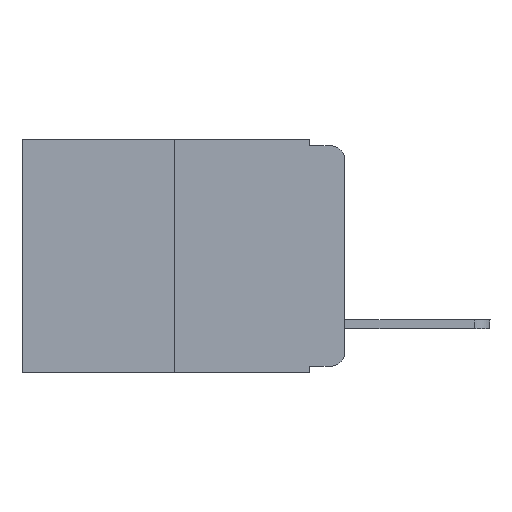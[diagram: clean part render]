
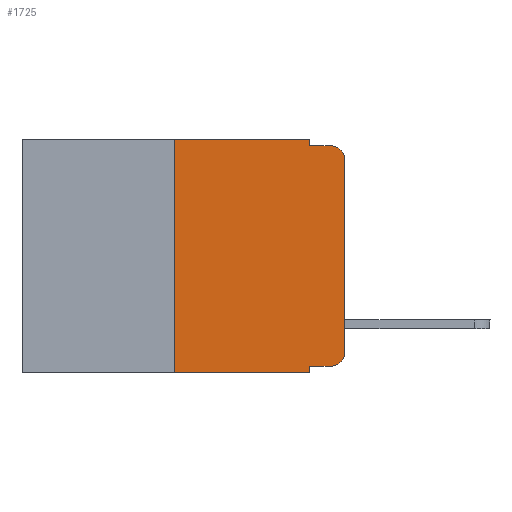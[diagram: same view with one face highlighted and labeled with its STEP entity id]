
A CAD part, left-side view. The second image highlights one B-rep face of the part: STEP entity #1725.
In plain terms, the highlighted planar face has unit normal (-1, 0, 0).
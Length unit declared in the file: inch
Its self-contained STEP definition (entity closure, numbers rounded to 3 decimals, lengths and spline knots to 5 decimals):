
#99 = EDGE_CURVE ( 'NONE', #9774, #3113, #4630, .T. ) ;
#187 = DIRECTION ( 'NONE',  ( 0., 0., 1. ) ) ;
#196 = DIRECTION ( 'NONE',  ( 0., 0., -1. ) ) ;
#486 = VECTOR ( 'NONE', #4476, 39.37008 ) ;
#588 = DIRECTION ( 'NONE',  ( 1., 0., 0. ) ) ;
#628 = DIRECTION ( 'NONE',  ( 0., -1., 0. ) ) ;
#664 = DIRECTION ( 'NONE',  ( 0., -1., 0. ) ) ;
#666 = ORIENTED_EDGE ( 'NONE', *, *, #4712, .T. ) ;
#962 = DIRECTION ( 'NONE',  ( -1., 0., 0. ) ) ;
#1232 = VECTOR ( 'NONE', #664, 39.37008 ) ;
#1253 = EDGE_CURVE ( 'NONE', #8522, #6959, #6556, .T. ) ;
#1318 = LINE ( 'NONE', #5188, #9555 ) ;
#1461 = VECTOR ( 'NONE', #628, 39.37008 ) ;
#1607 = VECTOR ( 'NONE', #8382, 39.37008 ) ;
#1681 = AXIS2_PLACEMENT_3D ( 'NONE', #4606, #588, #6903 ) ;
#1701 = EDGE_CURVE ( 'NONE', #6707, #2656, #3831, .T. ) ;
#1725 = ADVANCED_FACE ( 'NONE', ( #8867 ), #3811, .F. ) ;
#1744 = CARTESIAN_POINT ( 'NONE',  ( 0., 0.02, -0.03 ) ) ;
#2026 = ORIENTED_EDGE ( 'NONE', *, *, #7858, .F. ) ;
#2173 = VERTEX_POINT ( 'NONE', #7969 ) ;
#2255 = ORIENTED_EDGE ( 'NONE', *, *, #3252, .T. ) ;
#2523 = ORIENTED_EDGE ( 'NONE', *, *, #4235, .F. ) ;
#2622 = DIRECTION ( 'NONE',  ( 0., 0., -1. ) ) ;
#2656 = VERTEX_POINT ( 'NONE', #4890 ) ;
#2674 = VECTOR ( 'NONE', #4268, 39.37008 ) ;
#2708 = CARTESIAN_POINT ( 'NONE',  ( 0., 0.473, 0. ) ) ;
#2764 = EDGE_CURVE ( 'NONE', #6959, #4611, #4320, .T. ) ;
#3035 = ORIENTED_EDGE ( 'NONE', *, *, #1701, .T. ) ;
#3113 = VERTEX_POINT ( 'NONE', #9976 ) ;
#3252 = EDGE_CURVE ( 'NONE', #4224, #9774, #4693, .T. ) ;
#3350 = DIRECTION ( 'NONE',  ( 0., 0., -1. ) ) ;
#3436 = CARTESIAN_POINT ( 'NONE',  ( 0., 0.051, -0.333 ) ) ;
#3438 = AXIS2_PLACEMENT_3D ( 'NONE', #1744, #8988, #3350 ) ;
#3592 = ORIENTED_EDGE ( 'NONE', *, *, #9711, .T. ) ;
#3811 = PLANE ( 'NONE',  #1681 ) ;
#3831 = LINE ( 'NONE', #10121, #1232 ) ;
#3874 = ORIENTED_EDGE ( 'NONE', *, *, #1253, .F. ) ;
#4224 = VERTEX_POINT ( 'NONE', #3436 ) ;
#4235 = EDGE_CURVE ( 'NONE', #4224, #2656, #1318, .T. ) ;
#4268 = DIRECTION ( 'NONE',  ( 0., -1., 0. ) ) ;
#4320 = LINE ( 'NONE', #5224, #1607 ) ;
#4476 = DIRECTION ( 'NONE',  ( 0., -1., 0. ) ) ;
#4568 = DIRECTION ( 'NONE',  ( 0., 0., 1. ) ) ;
#4606 = CARTESIAN_POINT ( 'NONE',  ( 0., 0.473, 0. ) ) ;
#4611 = VERTEX_POINT ( 'NONE', #4865 ) ;
#4630 = CIRCLE ( 'NONE', #8134, 0.02 ) ;
#4637 = CARTESIAN_POINT ( 'NONE',  ( 0., 0., 0. ) ) ;
#4693 = LINE ( 'NONE', #6103, #1461 ) ;
#4712 = EDGE_CURVE ( 'NONE', #8580, #2173, #7694, .T. ) ;
#4865 = CARTESIAN_POINT ( 'NONE',  ( 0., 0.051, -0.01 ) ) ;
#4890 = CARTESIAN_POINT ( 'NONE',  ( 0., 0.051, -0.343 ) ) ;
#5188 = CARTESIAN_POINT ( 'NONE',  ( 0., 0.051, 0. ) ) ;
#5224 = CARTESIAN_POINT ( 'NONE',  ( 0., 0.051, 0. ) ) ;
#5352 = VECTOR ( 'NONE', #187, 39.37008 ) ;
#5365 = CARTESIAN_POINT ( 'NONE',  ( 0., 0.25, -0.343 ) ) ;
#6103 = CARTESIAN_POINT ( 'NONE',  ( 0., 0.051, -0.333 ) ) ;
#6229 = CARTESIAN_POINT ( 'NONE',  ( 0., 0.02, -0.333 ) ) ;
#6556 = LINE ( 'NONE', #2708, #2674 ) ;
#6707 = VERTEX_POINT ( 'NONE', #5365 ) ;
#6903 = DIRECTION ( 'NONE',  ( 0., 0., -1. ) ) ;
#6954 = CARTESIAN_POINT ( 'NONE',  ( 0., 0.051, -0.01 ) ) ;
#6959 = VERTEX_POINT ( 'NONE', #9571 ) ;
#7047 = CARTESIAN_POINT ( 'NONE',  ( 0., 0., -0.03 ) ) ;
#7324 = VECTOR ( 'NONE', #4568, 39.37008 ) ;
#7408 = CARTESIAN_POINT ( 'NONE',  ( 0., 0.25, 0. ) ) ;
#7552 = ORIENTED_EDGE ( 'NONE', *, *, #2764, .F. ) ;
#7636 = EDGE_CURVE ( 'NONE', #6707, #8522, #8114, .T. ) ;
#7694 = CIRCLE ( 'NONE', #3438, 0.02 ) ;
#7828 = CARTESIAN_POINT ( 'NONE',  ( 0., 0.25, 0. ) ) ;
#7858 = EDGE_CURVE ( 'NONE', #4611, #2173, #9817, .T. ) ;
#7969 = CARTESIAN_POINT ( 'NONE',  ( 0., 0.02, -0.01 ) ) ;
#8114 = LINE ( 'NONE', #7408, #5352 ) ;
#8123 = CARTESIAN_POINT ( 'NONE',  ( 0., 0.02, -0.313 ) ) ;
#8134 = AXIS2_PLACEMENT_3D ( 'NONE', #8123, #962, #196 ) ;
#8284 = EDGE_LOOP ( 'NONE', ( #3592, #666, #2026, #7552, #3874, #9654, #3035, #2523, #2255, #9341 ) ) ;
#8382 = DIRECTION ( 'NONE',  ( 0., 0., -1. ) ) ;
#8522 = VERTEX_POINT ( 'NONE', #7828 ) ;
#8580 = VERTEX_POINT ( 'NONE', #7047 ) ;
#8867 = FACE_OUTER_BOUND ( 'NONE', #8284, .T. ) ;
#8988 = DIRECTION ( 'NONE',  ( -1., 0., 0. ) ) ;
#9341 = ORIENTED_EDGE ( 'NONE', *, *, #99, .T. ) ;
#9555 = VECTOR ( 'NONE', #2622, 39.37008 ) ;
#9571 = CARTESIAN_POINT ( 'NONE',  ( 0., 0.051, 0. ) ) ;
#9654 = ORIENTED_EDGE ( 'NONE', *, *, #7636, .F. ) ;
#9711 = EDGE_CURVE ( 'NONE', #3113, #8580, #10279, .T. ) ;
#9774 = VERTEX_POINT ( 'NONE', #6229 ) ;
#9817 = LINE ( 'NONE', #6954, #486 ) ;
#9976 = CARTESIAN_POINT ( 'NONE',  ( 0., 0., -0.313 ) ) ;
#10121 = CARTESIAN_POINT ( 'NONE',  ( 0., 0.473, -0.343 ) ) ;
#10279 = LINE ( 'NONE', #4637, #7324 ) ;
